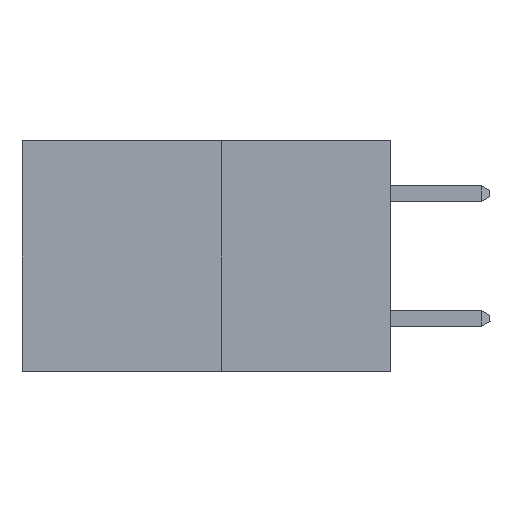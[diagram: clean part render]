
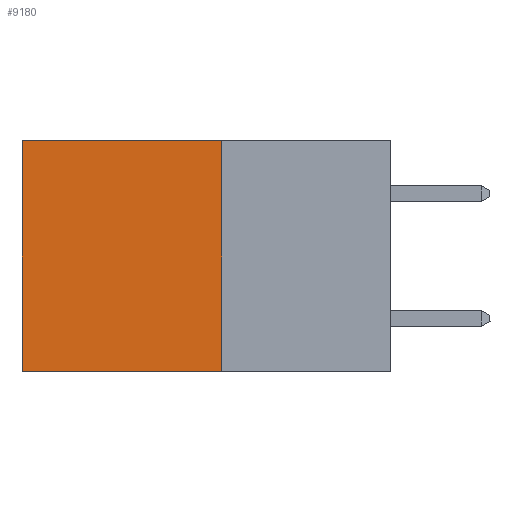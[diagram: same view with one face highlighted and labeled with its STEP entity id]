
A CAD part, left-side view. The second image highlights one B-rep face of the part: STEP entity #9180.
In plain terms, the highlighted planar face has unit normal (-1, 0, 0).
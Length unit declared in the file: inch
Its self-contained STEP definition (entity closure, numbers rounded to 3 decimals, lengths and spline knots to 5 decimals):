
#1154 = ORIENTED_EDGE ( 'NONE', *, *, #4402, .F. ) ;
#1534 = LINE ( 'NONE', #13376, #17382 ) ;
#1657 = VERTEX_POINT ( 'NONE', #6893 ) ;
#1989 = VERTEX_POINT ( 'NONE', #14191 ) ;
#2106 = EDGE_CURVE ( 'NONE', #21929, #1657, #1534, .T. ) ;
#2734 = VERTEX_POINT ( 'NONE', #23985 ) ;
#3220 = ORIENTED_EDGE ( 'NONE', *, *, #11823, .T. ) ;
#3612 = AXIS2_PLACEMENT_3D ( 'NONE', #27342, #26702, #26677 ) ;
#4402 = EDGE_CURVE ( 'NONE', #2734, #1989, #7214, .T. ) ;
#6893 = CARTESIAN_POINT ( 'NONE',  ( 0.277, 0.59, -0.37 ) ) ;
#7214 = LINE ( 'NONE', #15995, #22791 ) ;
#9180 = ADVANCED_FACE ( 'NONE', ( #24908 ), #27094, .F. ) ;
#11823 = EDGE_CURVE ( 'NONE', #2734, #21929, #23180, .T. ) ;
#12746 = CARTESIAN_POINT ( 'NONE',  ( 0.277, 0.59, 0. ) ) ;
#13239 = CARTESIAN_POINT ( 'NONE',  ( 0.277, 0.27, 0. ) ) ;
#13334 = DIRECTION ( 'NONE',  ( 0., 1., 0. ) ) ;
#13376 = CARTESIAN_POINT ( 'NONE',  ( 0.277, 0.59, -0.37 ) ) ;
#14191 = CARTESIAN_POINT ( 'NONE',  ( 0.277, 0.27, -0.37 ) ) ;
#14247 = EDGE_LOOP ( 'NONE', ( #23806, #27000, #1154, #3220 ) ) ;
#14411 = EDGE_CURVE ( 'NONE', #1989, #1657, #17018, .T. ) ;
#15183 = DIRECTION ( 'NONE',  ( 0., 0., -1. ) ) ;
#15995 = CARTESIAN_POINT ( 'NONE',  ( 0.277, 0.27, -0.37 ) ) ;
#17018 = LINE ( 'NONE', #25549, #27359 ) ;
#17382 = VECTOR ( 'NONE', #22983, 39.37008 ) ;
#17643 = VECTOR ( 'NONE', #13334, 39.37008 ) ;
#21929 = VERTEX_POINT ( 'NONE', #12746 ) ;
#22791 = VECTOR ( 'NONE', #15183, 39.37008 ) ;
#22983 = DIRECTION ( 'NONE',  ( 0., 0., -1. ) ) ;
#23180 = LINE ( 'NONE', #13239, #17643 ) ;
#23806 = ORIENTED_EDGE ( 'NONE', *, *, #2106, .T. ) ;
#23985 = CARTESIAN_POINT ( 'NONE',  ( 0.277, 0.27, 0. ) ) ;
#24908 = FACE_OUTER_BOUND ( 'NONE', #14247, .T. ) ;
#25494 = DIRECTION ( 'NONE',  ( 0., 1., 0. ) ) ;
#25549 = CARTESIAN_POINT ( 'NONE',  ( 0.277, 0.27, -0.37 ) ) ;
#26677 = DIRECTION ( 'NONE',  ( 0., 0., -1. ) ) ;
#26702 = DIRECTION ( 'NONE',  ( 1., 0., 0. ) ) ;
#27000 = ORIENTED_EDGE ( 'NONE', *, *, #14411, .F. ) ;
#27094 = PLANE ( 'NONE',  #3612 ) ;
#27342 = CARTESIAN_POINT ( 'NONE',  ( 0.277, 0.27, -0.37 ) ) ;
#27359 = VECTOR ( 'NONE', #25494, 39.37008 ) ;
